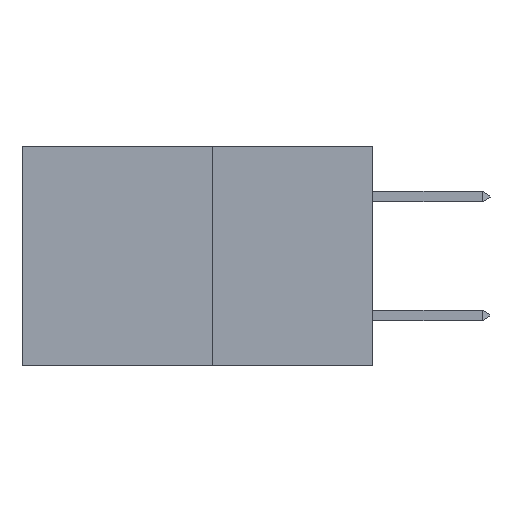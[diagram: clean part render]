
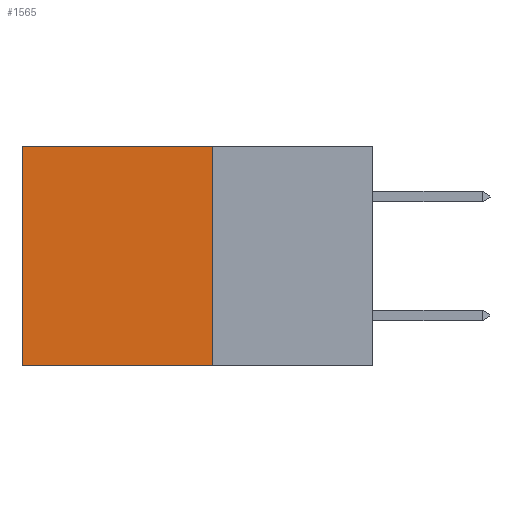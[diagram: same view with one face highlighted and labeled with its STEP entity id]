
A CAD part, left-side view. The second image highlights one B-rep face of the part: STEP entity #1565.
In plain terms, the highlighted planar face has unit normal (-1, 0, 0).
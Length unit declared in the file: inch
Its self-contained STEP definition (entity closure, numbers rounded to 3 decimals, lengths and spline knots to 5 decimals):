
#307 = CARTESIAN_POINT ( 'NONE',  ( 0.277, 0.27, -0.37 ) ) ;
#628 = AXIS2_PLACEMENT_3D ( 'NONE', #8378, #8013, #7443 ) ;
#1529 = VECTOR ( 'NONE', #4881, 39.37008 ) ;
#1565 = ADVANCED_FACE ( 'NONE', ( #1599 ), #9297, .F. ) ;
#1599 = FACE_OUTER_BOUND ( 'NONE', #5217, .T. ) ;
#1747 = VECTOR ( 'NONE', #5612, 39.37008 ) ;
#1821 = ORIENTED_EDGE ( 'NONE', *, *, #8274, .F. ) ;
#1996 = LINE ( 'NONE', #5587, #1529 ) ;
#2540 = ORIENTED_EDGE ( 'NONE', *, *, #3973, .T. ) ;
#2631 = VERTEX_POINT ( 'NONE', #9036 ) ;
#3189 = DIRECTION ( 'NONE',  ( 0., 0., -1. ) ) ;
#3274 = LINE ( 'NONE', #307, #1747 ) ;
#3961 = VERTEX_POINT ( 'NONE', #5066 ) ;
#3973 = EDGE_CURVE ( 'NONE', #3961, #2631, #5027, .T. ) ;
#4012 = ORIENTED_EDGE ( 'NONE', *, *, #7625, .T. ) ;
#4881 = DIRECTION ( 'NONE',  ( 0., 0., -1. ) ) ;
#4889 = DIRECTION ( 'NONE',  ( 0., 1., 0. ) ) ;
#5027 = LINE ( 'NONE', #5168, #8358 ) ;
#5066 = CARTESIAN_POINT ( 'NONE',  ( 0.277, 0.27, 0. ) ) ;
#5168 = CARTESIAN_POINT ( 'NONE',  ( 0.277, 0.27, 0. ) ) ;
#5217 = EDGE_LOOP ( 'NONE', ( #4012, #7842, #1821, #2540 ) ) ;
#5412 = LINE ( 'NONE', #6752, #8939 ) ;
#5587 = CARTESIAN_POINT ( 'NONE',  ( 0.277, 0.59, -0.37 ) ) ;
#5612 = DIRECTION ( 'NONE',  ( 0., 1., 0. ) ) ;
#6630 = VERTEX_POINT ( 'NONE', #8316 ) ;
#6752 = CARTESIAN_POINT ( 'NONE',  ( 0.277, 0.27, -0.37 ) ) ;
#7427 = VERTEX_POINT ( 'NONE', #8310 ) ;
#7443 = DIRECTION ( 'NONE',  ( 0., 0., -1. ) ) ;
#7625 = EDGE_CURVE ( 'NONE', #2631, #6630, #1996, .T. ) ;
#7681 = EDGE_CURVE ( 'NONE', #7427, #6630, #3274, .T. ) ;
#7842 = ORIENTED_EDGE ( 'NONE', *, *, #7681, .F. ) ;
#8013 = DIRECTION ( 'NONE',  ( 1., 0., 0. ) ) ;
#8274 = EDGE_CURVE ( 'NONE', #3961, #7427, #5412, .T. ) ;
#8310 = CARTESIAN_POINT ( 'NONE',  ( 0.277, 0.27, -0.37 ) ) ;
#8316 = CARTESIAN_POINT ( 'NONE',  ( 0.277, 0.59, -0.37 ) ) ;
#8358 = VECTOR ( 'NONE', #4889, 39.37008 ) ;
#8378 = CARTESIAN_POINT ( 'NONE',  ( 0.277, 0.27, -0.37 ) ) ;
#8939 = VECTOR ( 'NONE', #3189, 39.37008 ) ;
#9036 = CARTESIAN_POINT ( 'NONE',  ( 0.277, 0.59, 0. ) ) ;
#9297 = PLANE ( 'NONE',  #628 ) ;
